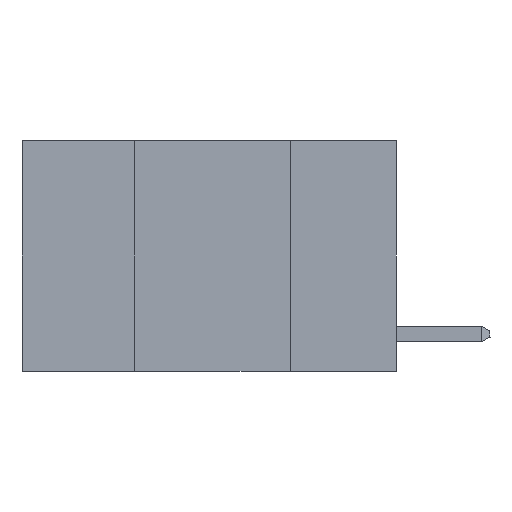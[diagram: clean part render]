
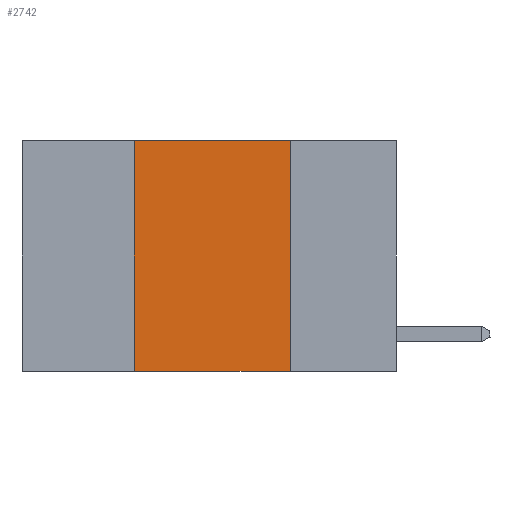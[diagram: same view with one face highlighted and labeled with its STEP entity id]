
A CAD part, left-side view. The second image highlights one B-rep face of the part: STEP entity #2742.
In plain terms, the highlighted planar face has unit normal (-1, 0, 0).
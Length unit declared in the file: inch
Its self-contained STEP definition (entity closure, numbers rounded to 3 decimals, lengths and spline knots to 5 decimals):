
#160 = DIRECTION ( 'NONE',  ( 0., 0., -1. ) ) ;
#594 = DIRECTION ( 'NONE',  ( 0., 0., -1. ) ) ;
#660 = ORIENTED_EDGE ( 'NONE', *, *, #10083, .F. ) ;
#952 = LINE ( 'NONE', #5389, #11114 ) ;
#2162 = VECTOR ( 'NONE', #6043, 39.37008 ) ;
#2309 = CARTESIAN_POINT ( 'NONE',  ( 0., 0.17, 0. ) ) ;
#2742 = ADVANCED_FACE ( 'NONE', ( #10129 ), #9454, .F. ) ;
#3096 = DIRECTION ( 'NONE',  ( 1., 0., 0. ) ) ;
#3571 = LINE ( 'NONE', #2309, #10925 ) ;
#3923 = CARTESIAN_POINT ( 'NONE',  ( 0., 0.42, -0.37 ) ) ;
#4514 = EDGE_CURVE ( 'NONE', #7695, #8819, #10057, .T. ) ;
#4642 = CARTESIAN_POINT ( 'NONE',  ( 0., 0.42, 0. ) ) ;
#4916 = CARTESIAN_POINT ( 'NONE',  ( 0., 0.6, 0. ) ) ;
#4989 = ORIENTED_EDGE ( 'NONE', *, *, #4514, .F. ) ;
#5049 = VERTEX_POINT ( 'NONE', #3923 ) ;
#5389 = CARTESIAN_POINT ( 'NONE',  ( 0., 0.6, -0.37 ) ) ;
#6043 = DIRECTION ( 'NONE',  ( 0., -1., 0. ) ) ;
#6944 = ORIENTED_EDGE ( 'NONE', *, *, #11449, .T. ) ;
#7223 = VECTOR ( 'NONE', #8207, 39.37008 ) ;
#7485 = CARTESIAN_POINT ( 'NONE',  ( 0., 0.6, 0. ) ) ;
#7695 = VERTEX_POINT ( 'NONE', #4642 ) ;
#7859 = CARTESIAN_POINT ( 'NONE',  ( 0., 0.17, 0. ) ) ;
#8142 = VERTEX_POINT ( 'NONE', #9952 ) ;
#8207 = DIRECTION ( 'NONE',  ( 0., 0., 1. ) ) ;
#8457 = ORIENTED_EDGE ( 'NONE', *, *, #11411, .F. ) ;
#8819 = VERTEX_POINT ( 'NONE', #7859 ) ;
#9152 = DIRECTION ( 'NONE',  ( 0., -1., 0. ) ) ;
#9304 = LINE ( 'NONE', #12606, #7223 ) ;
#9454 = PLANE ( 'NONE',  #11214 ) ;
#9952 = CARTESIAN_POINT ( 'NONE',  ( 0., 0.17, -0.37 ) ) ;
#10057 = LINE ( 'NONE', #4916, #2162 ) ;
#10083 = EDGE_CURVE ( 'NONE', #8819, #8142, #3571, .T. ) ;
#10129 = FACE_OUTER_BOUND ( 'NONE', #10575, .T. ) ;
#10575 = EDGE_LOOP ( 'NONE', ( #660, #4989, #8457, #6944 ) ) ;
#10925 = VECTOR ( 'NONE', #160, 39.37008 ) ;
#11114 = VECTOR ( 'NONE', #9152, 39.37008 ) ;
#11214 = AXIS2_PLACEMENT_3D ( 'NONE', #7485, #3096, #594 ) ;
#11411 = EDGE_CURVE ( 'NONE', #5049, #7695, #9304, .T. ) ;
#11449 = EDGE_CURVE ( 'NONE', #5049, #8142, #952, .T. ) ;
#12606 = CARTESIAN_POINT ( 'NONE',  ( 0., 0.42, 0. ) ) ;
